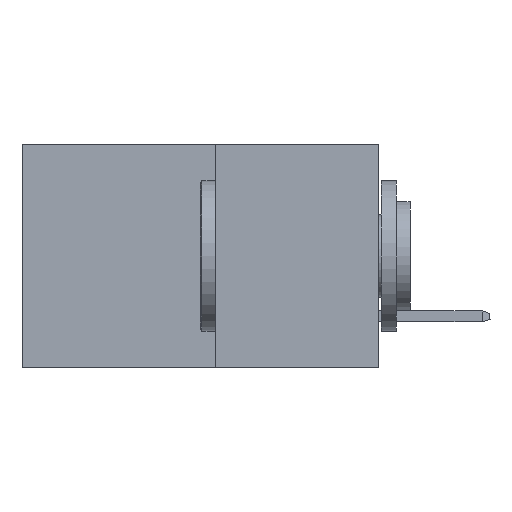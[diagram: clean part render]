
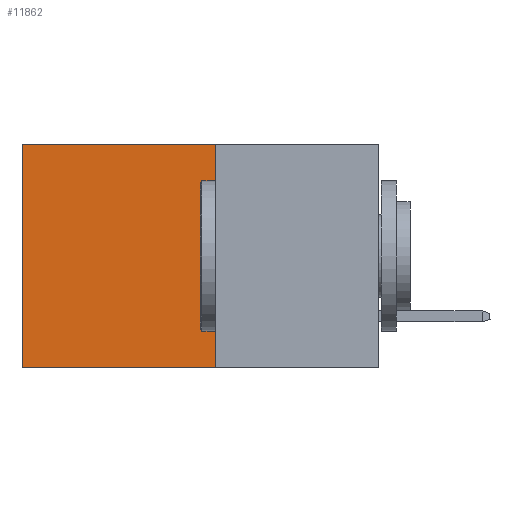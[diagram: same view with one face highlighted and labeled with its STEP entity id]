
A CAD part, left-side view. The second image highlights one B-rep face of the part: STEP entity #11862.
In plain terms, the highlighted planar face has unit normal (-1, 0, 0).
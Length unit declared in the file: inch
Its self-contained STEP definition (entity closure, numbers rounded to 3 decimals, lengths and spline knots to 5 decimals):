
#27 = DIRECTION ( 'NONE',  ( 0., 0., -1. ) ) ;
#1357 = EDGE_CURVE ( 'NONE', #14160, #11000, #16021, .T. ) ;
#1650 = ORIENTED_EDGE ( 'NONE', *, *, #5919, .F. ) ;
#2142 = EDGE_CURVE ( 'NONE', #13942, #4519, #17580, .T. ) ;
#2322 = CARTESIAN_POINT ( 'NONE',  ( 0.277, 0.59, -0.37 ) ) ;
#2644 = CARTESIAN_POINT ( 'NONE',  ( 0.277, 0.27, 0. ) ) ;
#4075 = CARTESIAN_POINT ( 'NONE',  ( 0.277, 0.59, -0.37 ) ) ;
#4411 = LINE ( 'NONE', #18027, #8743 ) ;
#4519 = VERTEX_POINT ( 'NONE', #13500 ) ;
#4749 = DIRECTION ( 'NONE',  ( 1., 0., 0. ) ) ;
#5701 = VECTOR ( 'NONE', #11833, 39.37008 ) ;
#5919 = EDGE_CURVE ( 'NONE', #4519, #11000, #4411, .T. ) ;
#6057 = CARTESIAN_POINT ( 'NONE',  ( 0.277, 0.59, 0. ) ) ;
#7402 = EDGE_LOOP ( 'NONE', ( #7990, #1650, #17517, #13592 ) ) ;
#7990 = ORIENTED_EDGE ( 'NONE', *, *, #1357, .T. ) ;
#8158 = FACE_OUTER_BOUND ( 'NONE', #7402, .T. ) ;
#8743 = VECTOR ( 'NONE', #17750, 39.37008 ) ;
#8985 = CARTESIAN_POINT ( 'NONE',  ( 0.277, 0.27, 0. ) ) ;
#9551 = CARTESIAN_POINT ( 'NONE',  ( 0.277, 0.27, -0.37 ) ) ;
#10598 = CARTESIAN_POINT ( 'NONE',  ( 0.277, 0.27, -0.37 ) ) ;
#10915 = VECTOR ( 'NONE', #13448, 39.37008 ) ;
#11000 = VERTEX_POINT ( 'NONE', #4075 ) ;
#11833 = DIRECTION ( 'NONE',  ( 0., 0., -1. ) ) ;
#11862 = ADVANCED_FACE ( 'NONE', ( #8158 ), #13555, .F. ) ;
#13448 = DIRECTION ( 'NONE',  ( 0., 1., 0. ) ) ;
#13500 = CARTESIAN_POINT ( 'NONE',  ( 0.277, 0.27, -0.37 ) ) ;
#13555 = PLANE ( 'NONE',  #14922 ) ;
#13592 = ORIENTED_EDGE ( 'NONE', *, *, #13621, .T. ) ;
#13621 = EDGE_CURVE ( 'NONE', #13942, #14160, #15271, .T. ) ;
#13744 = VECTOR ( 'NONE', #27, 39.37008 ) ;
#13942 = VERTEX_POINT ( 'NONE', #2644 ) ;
#14160 = VERTEX_POINT ( 'NONE', #6057 ) ;
#14922 = AXIS2_PLACEMENT_3D ( 'NONE', #10598, #4749, #15039 ) ;
#15039 = DIRECTION ( 'NONE',  ( 0., 0., -1. ) ) ;
#15271 = LINE ( 'NONE', #8985, #10915 ) ;
#16021 = LINE ( 'NONE', #2322, #5701 ) ;
#17517 = ORIENTED_EDGE ( 'NONE', *, *, #2142, .F. ) ;
#17580 = LINE ( 'NONE', #9551, #13744 ) ;
#17750 = DIRECTION ( 'NONE',  ( 0., 1., 0. ) ) ;
#18027 = CARTESIAN_POINT ( 'NONE',  ( 0.277, 0.27, -0.37 ) ) ;
